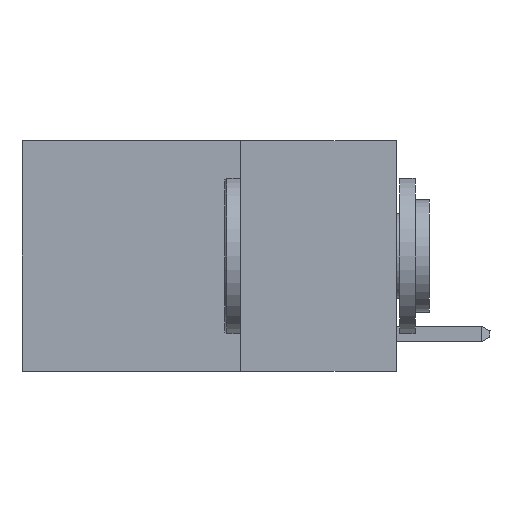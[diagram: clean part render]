
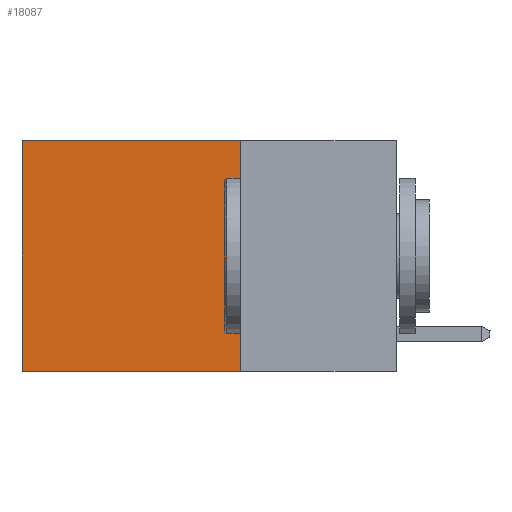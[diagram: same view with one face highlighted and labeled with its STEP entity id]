
A CAD part, left-side view. The second image highlights one B-rep face of the part: STEP entity #18087.
In plain terms, the highlighted planar face has unit normal (-1, 0, 0).
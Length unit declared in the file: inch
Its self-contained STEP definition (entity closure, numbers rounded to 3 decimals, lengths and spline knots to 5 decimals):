
#419 = LINE ( 'NONE', #21805, #4954 ) ;
#625 = VERTEX_POINT ( 'NONE', #17084 ) ;
#663 = CARTESIAN_POINT ( 'NONE',  ( 0.2625, 0.25, 0. ) ) ;
#811 = EDGE_CURVE ( 'NONE', #27072, #10196, #419, .T. ) ;
#2537 = VECTOR ( 'NONE', #7372, 39.37008 ) ;
#3863 = AXIS2_PLACEMENT_3D ( 'NONE', #5030, #13697, #22435 ) ;
#4249 = ORIENTED_EDGE ( 'NONE', *, *, #17614, .T. ) ;
#4954 = VECTOR ( 'NONE', #6657, 39.37008 ) ;
#5030 = CARTESIAN_POINT ( 'NONE',  ( 0.2625, 0.25, 0. ) ) ;
#6657 = DIRECTION ( 'NONE',  ( 0., 1., 0. ) ) ;
#7332 = DIRECTION ( 'NONE',  ( 0., 0., -1. ) ) ;
#7372 = DIRECTION ( 'NONE',  ( 0., 1., 0. ) ) ;
#7926 = ORIENTED_EDGE ( 'NONE', *, *, #15564, .F. ) ;
#9027 = CARTESIAN_POINT ( 'NONE',  ( 0.2625, 0.6, -0.37 ) ) ;
#9319 = DIRECTION ( 'NONE',  ( 0., 0., -1. ) ) ;
#9368 = LINE ( 'NONE', #24221, #2537 ) ;
#9422 = ORIENTED_EDGE ( 'NONE', *, *, #811, .F. ) ;
#10196 = VERTEX_POINT ( 'NONE', #9027 ) ;
#11743 = LINE ( 'NONE', #663, #17994 ) ;
#13020 = EDGE_LOOP ( 'NONE', ( #4249, #9422, #7926, #15947 ) ) ;
#13697 = DIRECTION ( 'NONE',  ( 1., 0., 0. ) ) ;
#15564 = EDGE_CURVE ( 'NONE', #25714, #27072, #11743, .T. ) ;
#15864 = PLANE ( 'NONE',  #3863 ) ;
#15903 = CARTESIAN_POINT ( 'NONE',  ( 0.2625, 0.6, 0. ) ) ;
#15947 = ORIENTED_EDGE ( 'NONE', *, *, #23974, .T. ) ;
#16054 = CARTESIAN_POINT ( 'NONE',  ( 0.2625, 0.25, 0. ) ) ;
#17084 = CARTESIAN_POINT ( 'NONE',  ( 0.2625, 0.6, 0. ) ) ;
#17614 = EDGE_CURVE ( 'NONE', #625, #10196, #17897, .T. ) ;
#17897 = LINE ( 'NONE', #15903, #26158 ) ;
#17994 = VECTOR ( 'NONE', #9319, 39.37008 ) ;
#18087 = ADVANCED_FACE ( 'NONE', ( #26712 ), #15864, .F. ) ;
#20389 = CARTESIAN_POINT ( 'NONE',  ( 0.2625, 0.25, -0.37 ) ) ;
#21805 = CARTESIAN_POINT ( 'NONE',  ( 0.2625, 0.25, -0.37 ) ) ;
#22435 = DIRECTION ( 'NONE',  ( 0., 0., -1. ) ) ;
#23974 = EDGE_CURVE ( 'NONE', #25714, #625, #9368, .T. ) ;
#24221 = CARTESIAN_POINT ( 'NONE',  ( 0.2625, 0.25, 0. ) ) ;
#25714 = VERTEX_POINT ( 'NONE', #16054 ) ;
#26158 = VECTOR ( 'NONE', #7332, 39.37008 ) ;
#26712 = FACE_OUTER_BOUND ( 'NONE', #13020, .T. ) ;
#27072 = VERTEX_POINT ( 'NONE', #20389 ) ;
